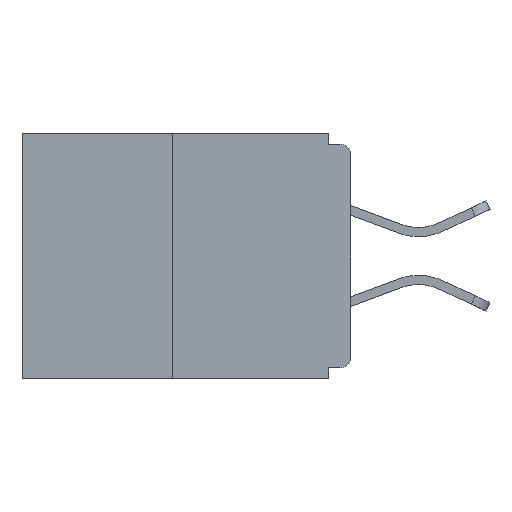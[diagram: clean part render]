
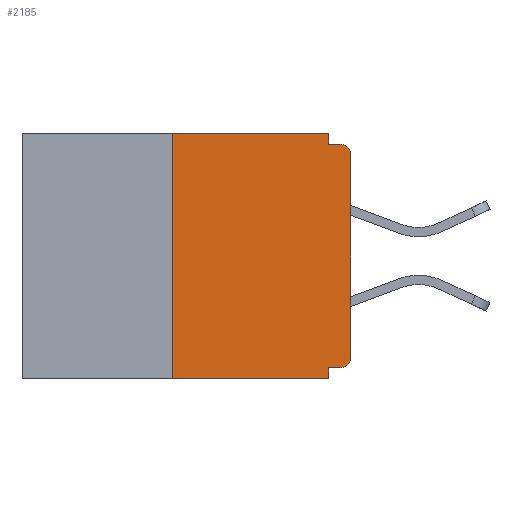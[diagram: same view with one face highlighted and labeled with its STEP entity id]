
A CAD part, left-side view. The second image highlights one B-rep face of the part: STEP entity #2185.
In plain terms, the highlighted planar face has unit normal (-1, 0, 0).
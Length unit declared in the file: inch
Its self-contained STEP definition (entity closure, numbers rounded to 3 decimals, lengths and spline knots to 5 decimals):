
#301 = VERTEX_POINT ( 'NONE', #2071 ) ;
#365 = CARTESIAN_POINT ( 'NONE',  ( 0., 0.46, 0. ) ) ;
#743 = DIRECTION ( 'NONE',  ( -1., 0., 0. ) ) ;
#820 = EDGE_CURVE ( 'NONE', #301, #10337, #13697, .T. ) ;
#998 = ORIENTED_EDGE ( 'NONE', *, *, #11209, .F. ) ;
#1353 = VERTEX_POINT ( 'NONE', #9577 ) ;
#1568 = CARTESIAN_POINT ( 'NONE',  ( 0., 0.031, 0. ) ) ;
#1569 = DIRECTION ( 'NONE',  ( 0., -1., 0. ) ) ;
#1883 = CARTESIAN_POINT ( 'NONE',  ( 0., 0.015, -0.015 ) ) ;
#1975 = DIRECTION ( 'NONE',  ( 0., 1., 0. ) ) ;
#2071 = CARTESIAN_POINT ( 'NONE',  ( 0., 0.031, 0. ) ) ;
#2100 = ORIENTED_EDGE ( 'NONE', *, *, #2894, .F. ) ;
#2185 = ADVANCED_FACE ( 'NONE', ( #4520 ), #6162, .F. ) ;
#2304 = ORIENTED_EDGE ( 'NONE', *, *, #11101, .T. ) ;
#2340 = VECTOR ( 'NONE', #6198, 39.37008 ) ;
#2602 = CIRCLE ( 'NONE', #11979, 0.015 ) ;
#2704 = LINE ( 'NONE', #5136, #5378 ) ;
#2871 = CARTESIAN_POINT ( 'NONE',  ( 0., 0.031, -0.328 ) ) ;
#2894 = EDGE_CURVE ( 'NONE', #10337, #6097, #7038, .T. ) ;
#3017 = EDGE_CURVE ( 'NONE', #14295, #1353, #10492, .T. ) ;
#3083 = DIRECTION ( 'NONE',  ( -1., 0., 0. ) ) ;
#4078 = DIRECTION ( 'NONE',  ( 0., 0., -1. ) ) ;
#4279 = VERTEX_POINT ( 'NONE', #2871 ) ;
#4318 = VECTOR ( 'NONE', #11308, 39.37008 ) ;
#4520 = FACE_OUTER_BOUND ( 'NONE', #12666, .T. ) ;
#5022 = LINE ( 'NONE', #10843, #8340 ) ;
#5136 = CARTESIAN_POINT ( 'NONE',  ( 0., 0.46, 0. ) ) ;
#5314 = CARTESIAN_POINT ( 'NONE',  ( 0., 0., -0.03 ) ) ;
#5367 = LINE ( 'NONE', #9654, #2340 ) ;
#5378 = VECTOR ( 'NONE', #8577, 39.37008 ) ;
#5420 = ORIENTED_EDGE ( 'NONE', *, *, #3017, .F. ) ;
#5899 = CARTESIAN_POINT ( 'NONE',  ( 0., 0., -0.015 ) ) ;
#6097 = VERTEX_POINT ( 'NONE', #1883 ) ;
#6162 = PLANE ( 'NONE',  #7789 ) ;
#6198 = DIRECTION ( 'NONE',  ( 0., 0., -1. ) ) ;
#6201 = DIRECTION ( 'NONE',  ( 0., 0., 1. ) ) ;
#6732 = CARTESIAN_POINT ( 'NONE',  ( 0., 0.25, 0. ) ) ;
#7038 = LINE ( 'NONE', #5899, #11973 ) ;
#7269 = EDGE_CURVE ( 'NONE', #14295, #8722, #7662, .T. ) ;
#7662 = LINE ( 'NONE', #8481, #11315 ) ;
#7699 = DIRECTION ( 'NONE',  ( 0., 0., -1. ) ) ;
#7759 = CARTESIAN_POINT ( 'NONE',  ( 0., 0., -0.313 ) ) ;
#7789 = AXIS2_PLACEMENT_3D ( 'NONE', #365, #8444, #10662 ) ;
#8046 = ORIENTED_EDGE ( 'NONE', *, *, #11176, .T. ) ;
#8091 = EDGE_CURVE ( 'NONE', #9067, #6097, #2602, .T. ) ;
#8321 = AXIS2_PLACEMENT_3D ( 'NONE', #14731, #3083, #7699 ) ;
#8340 = VECTOR ( 'NONE', #6201, 39.37008 ) ;
#8444 = DIRECTION ( 'NONE',  ( 1., 0., 0. ) ) ;
#8481 = CARTESIAN_POINT ( 'NONE',  ( 0., 0.46, -0.343 ) ) ;
#8577 = DIRECTION ( 'NONE',  ( 0., -1., 0. ) ) ;
#8722 = VERTEX_POINT ( 'NONE', #13770 ) ;
#9067 = VERTEX_POINT ( 'NONE', #5314 ) ;
#9354 = CARTESIAN_POINT ( 'NONE',  ( 0., 0.25, -0.343 ) ) ;
#9577 = CARTESIAN_POINT ( 'NONE',  ( 0., 0.25, 0. ) ) ;
#9654 = CARTESIAN_POINT ( 'NONE',  ( 0., 0.031, -0.343 ) ) ;
#9877 = DIRECTION ( 'NONE',  ( 0., -1., 0. ) ) ;
#9969 = VERTEX_POINT ( 'NONE', #7759 ) ;
#10003 = EDGE_CURVE ( 'NONE', #11267, #4279, #12711, .T. ) ;
#10337 = VERTEX_POINT ( 'NONE', #12788 ) ;
#10338 = VECTOR ( 'NONE', #1975, 39.37008 ) ;
#10492 = LINE ( 'NONE', #6732, #4318 ) ;
#10662 = DIRECTION ( 'NONE',  ( 0., 0., -1. ) ) ;
#10843 = CARTESIAN_POINT ( 'NONE',  ( 0., 0., 0. ) ) ;
#11101 = EDGE_CURVE ( 'NONE', #11267, #9969, #11788, .T. ) ;
#11176 = EDGE_CURVE ( 'NONE', #9969, #9067, #5022, .T. ) ;
#11178 = CARTESIAN_POINT ( 'NONE',  ( 0., 0., -0.328 ) ) ;
#11209 = EDGE_CURVE ( 'NONE', #1353, #301, #2704, .T. ) ;
#11267 = VERTEX_POINT ( 'NONE', #12281 ) ;
#11308 = DIRECTION ( 'NONE',  ( 0., 0., 1. ) ) ;
#11315 = VECTOR ( 'NONE', #1569, 39.37008 ) ;
#11788 = CIRCLE ( 'NONE', #8321, 0.015 ) ;
#11973 = VECTOR ( 'NONE', #9877, 39.37008 ) ;
#11979 = AXIS2_PLACEMENT_3D ( 'NONE', #14874, #743, #4078 ) ;
#12281 = CARTESIAN_POINT ( 'NONE',  ( 0., 0.015, -0.328 ) ) ;
#12421 = VECTOR ( 'NONE', #14216, 39.37008 ) ;
#12537 = ORIENTED_EDGE ( 'NONE', *, *, #820, .F. ) ;
#12666 = EDGE_LOOP ( 'NONE', ( #998, #5420, #14280, #12967, #13236, #2304, #8046, #14086, #2100, #12537 ) ) ;
#12711 = LINE ( 'NONE', #11178, #10338 ) ;
#12788 = CARTESIAN_POINT ( 'NONE',  ( 0., 0.031, -0.015 ) ) ;
#12967 = ORIENTED_EDGE ( 'NONE', *, *, #14562, .F. ) ;
#13236 = ORIENTED_EDGE ( 'NONE', *, *, #10003, .F. ) ;
#13697 = LINE ( 'NONE', #1568, #12421 ) ;
#13770 = CARTESIAN_POINT ( 'NONE',  ( 0., 0.031, -0.343 ) ) ;
#14086 = ORIENTED_EDGE ( 'NONE', *, *, #8091, .T. ) ;
#14216 = DIRECTION ( 'NONE',  ( 0., 0., -1. ) ) ;
#14280 = ORIENTED_EDGE ( 'NONE', *, *, #7269, .T. ) ;
#14295 = VERTEX_POINT ( 'NONE', #9354 ) ;
#14562 = EDGE_CURVE ( 'NONE', #4279, #8722, #5367, .T. ) ;
#14731 = CARTESIAN_POINT ( 'NONE',  ( 0., 0.015, -0.313 ) ) ;
#14874 = CARTESIAN_POINT ( 'NONE',  ( 0., 0.015, -0.03 ) ) ;
